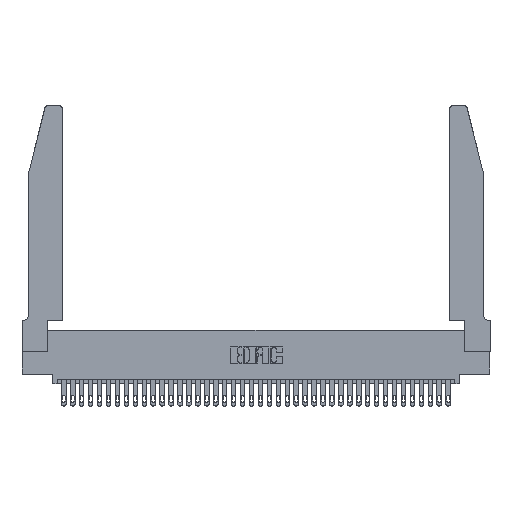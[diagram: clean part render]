
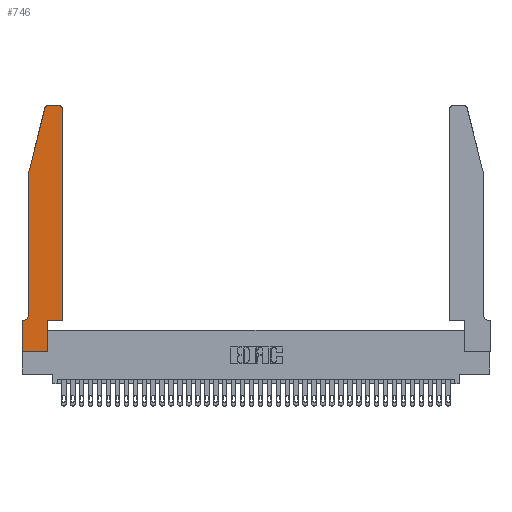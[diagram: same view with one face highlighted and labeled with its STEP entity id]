
A CAD part, top view. The second image highlights one B-rep face of the part: STEP entity #746.
In plain terms, the highlighted planar face has unit normal (0, 0, 1).
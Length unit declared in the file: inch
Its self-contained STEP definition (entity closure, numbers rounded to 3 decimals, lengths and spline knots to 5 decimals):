
#91 = VERTEX_POINT ( 'NONE', #24200 ) ;
#121 = ORIENTED_EDGE ( 'NONE', *, *, #3525, .T. ) ;
#301 = CARTESIAN_POINT ( 'NONE',  ( 0.0055, 0.42, 0.37 ) ) ;
#302 = EDGE_CURVE ( 'NONE', #16488, #21574, #4221, .T. ) ;
#356 = AXIS2_PLACEMENT_3D ( 'NONE', #38017, #7915, #20645 ) ;
#410 = CARTESIAN_POINT ( 'NONE',  ( 0.0755, 2., 0.37 ) ) ;
#746 = ADVANCED_FACE ( 'NONE', ( #6076 ), #25940, .T. ) ;
#919 = ORIENTED_EDGE ( 'NONE', *, *, #36220, .T. ) ;
#1149 = ORIENTED_EDGE ( 'NONE', *, *, #15967, .T. ) ;
#1242 = VERTEX_POINT ( 'NONE', #38084 ) ;
#2329 = DIRECTION ( 'NONE',  ( -1., 0., 0. ) ) ;
#2503 = EDGE_CURVE ( 'NONE', #22275, #2766, #28046, .T. ) ;
#2766 = VERTEX_POINT ( 'NONE', #17575 ) ;
#3304 = CARTESIAN_POINT ( 'NONE',  ( 0.4505, 2.72, 0.37 ) ) ;
#3525 = EDGE_CURVE ( 'NONE', #1242, #15845, #20451, .T. ) ;
#4204 = AXIS2_PLACEMENT_3D ( 'NONE', #31322, #22301, #31463 ) ;
#4221 = LINE ( 'NONE', #8798, #30588 ) ;
#5029 = DIRECTION ( 'NONE',  ( 1., 0., 0. ) ) ;
#5349 = CARTESIAN_POINT ( 'NONE',  ( 0.0755, 0.35, 0.37 ) ) ;
#5426 = CARTESIAN_POINT ( 'NONE',  ( 0., 0.35, 0.37 ) ) ;
#5771 = ORIENTED_EDGE ( 'NONE', *, *, #18354, .T. ) ;
#6076 = FACE_OUTER_BOUND ( 'NONE', #17309, .T. ) ;
#6161 = EDGE_CURVE ( 'NONE', #15845, #8153, #38789, .T. ) ;
#6176 = CARTESIAN_POINT ( 'NONE',  ( 0., 0., 0.37 ) ) ;
#6287 = VECTOR ( 'NONE', #2329, 39.37008 ) ;
#6526 = VECTOR ( 'NONE', #11298, 39.37008 ) ;
#6901 = ORIENTED_EDGE ( 'NONE', *, *, #6161, .T. ) ;
#7189 = ORIENTED_EDGE ( 'NONE', *, *, #24387, .T. ) ;
#7915 = DIRECTION ( 'NONE',  ( 0., 0., 1. ) ) ;
#8153 = VERTEX_POINT ( 'NONE', #26579 ) ;
#8248 = VECTOR ( 'NONE', #18233, 39.37008 ) ;
#8798 = CARTESIAN_POINT ( 'NONE',  ( 0.0755, 2., 0.37 ) ) ;
#8831 = EDGE_CURVE ( 'NONE', #36370, #32346, #16398, .T. ) ;
#9448 = LINE ( 'NONE', #26008, #38277 ) ;
#9573 = EDGE_CURVE ( 'NONE', #91, #22275, #22507, .T. ) ;
#9812 = CARTESIAN_POINT ( 'NONE',  ( 0., 0.35, 0.37 ) ) ;
#11298 = DIRECTION ( 'NONE',  ( 0., 1., 0. ) ) ;
#11799 = VERTEX_POINT ( 'NONE', #17228 ) ;
#11832 = CIRCLE ( 'NONE', #356, 0.03 ) ;
#12516 = DIRECTION ( 'NONE',  ( 1., 0., 0. ) ) ;
#13772 = DIRECTION ( 'NONE',  ( 0., 1., 0. ) ) ;
#14486 = CARTESIAN_POINT ( 'NONE',  ( 0.2865, 0.35, 0.37 ) ) ;
#15845 = VERTEX_POINT ( 'NONE', #9812 ) ;
#15967 = EDGE_CURVE ( 'NONE', #32346, #38977, #22250, .T. ) ;
#16398 = CIRCLE ( 'NONE', #4204, 0.03 ) ;
#16488 = VERTEX_POINT ( 'NONE', #35128 ) ;
#17228 = CARTESIAN_POINT ( 'NONE',  ( 0.0755, 0.42, 0.37 ) ) ;
#17309 = EDGE_LOOP ( 'NONE', ( #1149, #5771, #30976, #919, #20418, #121, #6901, #7189, #31252, #28730, #17869, #28071 ) ) ;
#17506 = VECTOR ( 'NONE', #21247, 39.37008 ) ;
#17575 = CARTESIAN_POINT ( 'NONE',  ( 0.4505, 0.35, 0.37 ) ) ;
#17869 = ORIENTED_EDGE ( 'NONE', *, *, #17909, .T. ) ;
#17909 = EDGE_CURVE ( 'NONE', #2766, #36370, #9448, .T. ) ;
#18233 = DIRECTION ( 'NONE',  ( 1., 0., 0. ) ) ;
#18354 = EDGE_CURVE ( 'NONE', #38977, #16488, #11832, .T. ) ;
#20418 = ORIENTED_EDGE ( 'NONE', *, *, #31485, .T. ) ;
#20451 = LINE ( 'NONE', #5349, #21825 ) ;
#20507 = CIRCLE ( 'NONE', #38881, 0.07 ) ;
#20645 = DIRECTION ( 'NONE',  ( 1., 0., 0. ) ) ;
#21247 = DIRECTION ( 'NONE',  ( 0., -1., 0. ) ) ;
#21376 = DIRECTION ( 'NONE',  ( 0., 0., -1. ) ) ;
#21574 = VERTEX_POINT ( 'NONE', #410 ) ;
#21825 = VECTOR ( 'NONE', #29425, 39.37008 ) ;
#22250 = LINE ( 'NONE', #26965, #6287 ) ;
#22275 = VERTEX_POINT ( 'NONE', #14486 ) ;
#22301 = DIRECTION ( 'NONE',  ( 0., 0., 1. ) ) ;
#22507 = LINE ( 'NONE', #32681, #6526 ) ;
#24200 = CARTESIAN_POINT ( 'NONE',  ( 0.2865, 0., 0.37 ) ) ;
#24387 = EDGE_CURVE ( 'NONE', #8153, #91, #32033, .T. ) ;
#25940 = PLANE ( 'NONE',  #31768 ) ;
#26008 = CARTESIAN_POINT ( 'NONE',  ( 0.4505, 0.35, 0.37 ) ) ;
#26579 = CARTESIAN_POINT ( 'NONE',  ( 0., 0., 0.37 ) ) ;
#26747 = DIRECTION ( 'NONE',  ( 0., -1., 0. ) ) ;
#26821 = DIRECTION ( 'NONE',  ( -0.239, -0.971, 0. ) ) ;
#26965 = CARTESIAN_POINT ( 'NONE',  ( 0.2605, 2.75, 0.37 ) ) ;
#27135 = CARTESIAN_POINT ( 'NONE',  ( 0.0755, 2., 0.37 ) ) ;
#28046 = LINE ( 'NONE', #38898, #8248 ) ;
#28071 = ORIENTED_EDGE ( 'NONE', *, *, #8831, .T. ) ;
#28730 = ORIENTED_EDGE ( 'NONE', *, *, #2503, .T. ) ;
#29256 = DIRECTION ( 'NONE',  ( 0., 0., 1. ) ) ;
#29425 = DIRECTION ( 'NONE',  ( -1., 0., 0. ) ) ;
#30588 = VECTOR ( 'NONE', #26821, 39.37008 ) ;
#30705 = CARTESIAN_POINT ( 'NONE',  ( 0., 0., 0.37 ) ) ;
#30976 = ORIENTED_EDGE ( 'NONE', *, *, #302, .T. ) ;
#31252 = ORIENTED_EDGE ( 'NONE', *, *, #9573, .T. ) ;
#31322 = CARTESIAN_POINT ( 'NONE',  ( 0.4205, 2.72, 0.37 ) ) ;
#31463 = DIRECTION ( 'NONE',  ( 1., 0., 0. ) ) ;
#31485 = EDGE_CURVE ( 'NONE', #11799, #1242, #20507, .T. ) ;
#31768 = AXIS2_PLACEMENT_3D ( 'NONE', #5426, #29256, #5029 ) ;
#32033 = LINE ( 'NONE', #30705, #33464 ) ;
#32225 = VECTOR ( 'NONE', #26747, 39.37008 ) ;
#32346 = VERTEX_POINT ( 'NONE', #32630 ) ;
#32550 = CARTESIAN_POINT ( 'NONE',  ( 0.284, 2.75, 0.37 ) ) ;
#32630 = CARTESIAN_POINT ( 'NONE',  ( 0.4205, 2.75, 0.37 ) ) ;
#32681 = CARTESIAN_POINT ( 'NONE',  ( 0.2865, 0.35, 0.37 ) ) ;
#33464 = VECTOR ( 'NONE', #12516, 39.37008 ) ;
#35071 = LINE ( 'NONE', #27135, #32225 ) ;
#35128 = CARTESIAN_POINT ( 'NONE',  ( 0.25487, 2.72718, 0.37 ) ) ;
#36220 = EDGE_CURVE ( 'NONE', #21574, #11799, #35071, .T. ) ;
#36370 = VERTEX_POINT ( 'NONE', #3304 ) ;
#36888 = DIRECTION ( 'NONE',  ( -1., 0., 0. ) ) ;
#38017 = CARTESIAN_POINT ( 'NONE',  ( 0.284, 2.72, 0.37 ) ) ;
#38084 = CARTESIAN_POINT ( 'NONE',  ( 0.0055, 0.35, 0.37 ) ) ;
#38277 = VECTOR ( 'NONE', #13772, 39.37008 ) ;
#38789 = LINE ( 'NONE', #6176, #17506 ) ;
#38881 = AXIS2_PLACEMENT_3D ( 'NONE', #301, #21376, #36888 ) ;
#38898 = CARTESIAN_POINT ( 'NONE',  ( 0.4505, 0.35, 0.37 ) ) ;
#38977 = VERTEX_POINT ( 'NONE', #32550 ) ;
